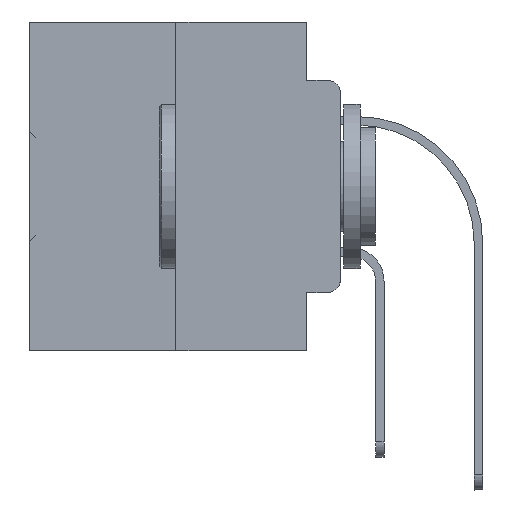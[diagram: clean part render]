
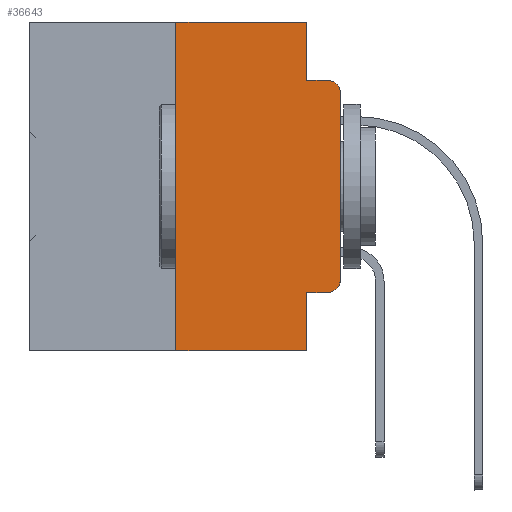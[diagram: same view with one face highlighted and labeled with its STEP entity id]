
A CAD part, left-side view. The second image highlights one B-rep face of the part: STEP entity #36643.
In plain terms, the highlighted planar face has unit normal (-1, 0, 0).
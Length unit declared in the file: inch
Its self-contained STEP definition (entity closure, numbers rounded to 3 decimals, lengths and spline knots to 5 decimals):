
#1444 = DIRECTION ( 'NONE',  ( 0., 0., -1. ) ) ;
#1654 = LINE ( 'NONE', #26141, #11457 ) ;
#1697 = CARTESIAN_POINT ( 'NONE',  ( 0., 0.473, 0. ) ) ;
#1804 = ORIENTED_EDGE ( 'NONE', *, *, #2692, .T. ) ;
#1989 = ORIENTED_EDGE ( 'NONE', *, *, #2322, .F. ) ;
#2322 = EDGE_CURVE ( 'NONE', #38294, #11469, #15991, .T. ) ;
#2692 = EDGE_CURVE ( 'NONE', #21018, #4290, #6643, .T. ) ;
#2758 = EDGE_CURVE ( 'NONE', #32369, #4290, #17079, .T. ) ;
#2951 = ORIENTED_EDGE ( 'NONE', *, *, #16692, .T. ) ;
#3166 = AXIS2_PLACEMENT_3D ( 'NONE', #30607, #5493, #18064 ) ;
#3219 = CARTESIAN_POINT ( 'NONE',  ( 0., 0., 0. ) ) ;
#3362 = CARTESIAN_POINT ( 'NONE',  ( 0., 0.473, -0.5 ) ) ;
#3396 = VECTOR ( 'NONE', #21791, 39.37008 ) ;
#3532 = EDGE_CURVE ( 'NONE', #37398, #5097, #38637, .T. ) ;
#3602 = VERTEX_POINT ( 'NONE', #37569 ) ;
#4290 = VERTEX_POINT ( 'NONE', #4984 ) ;
#4327 = DIRECTION ( 'NONE',  ( 0., -1., 0. ) ) ;
#4838 = ORIENTED_EDGE ( 'NONE', *, *, #2758, .F. ) ;
#4984 = CARTESIAN_POINT ( 'NONE',  ( 0., 0.051, -0.5 ) ) ;
#5050 = VECTOR ( 'NONE', #28550, 39.37008 ) ;
#5097 = VERTEX_POINT ( 'NONE', #39298 ) ;
#5493 = DIRECTION ( 'NONE',  ( -1., 0., 0. ) ) ;
#6643 = LINE ( 'NONE', #3362, #22549 ) ;
#7458 = DIRECTION ( 'NONE',  ( -1., 0., 0. ) ) ;
#8675 = VECTOR ( 'NONE', #28389, 39.37008 ) ;
#9003 = ORIENTED_EDGE ( 'NONE', *, *, #27369, .F. ) ;
#9231 = ORIENTED_EDGE ( 'NONE', *, *, #3532, .T. ) ;
#10164 = AXIS2_PLACEMENT_3D ( 'NONE', #32738, #7458, #32967 ) ;
#10305 = CARTESIAN_POINT ( 'NONE',  ( 0., 0., -0.1085 ) ) ;
#10973 = FACE_OUTER_BOUND ( 'NONE', #37685, .T. ) ;
#11457 = VECTOR ( 'NONE', #4327, 39.37008 ) ;
#11469 = VERTEX_POINT ( 'NONE', #20327 ) ;
#11607 = DIRECTION ( 'NONE',  ( 0., 0., -1. ) ) ;
#12340 = LINE ( 'NONE', #37397, #3396 ) ;
#12501 = LINE ( 'NONE', #3219, #33699 ) ;
#12686 = EDGE_CURVE ( 'NONE', #3602, #40446, #32276, .T. ) ;
#14261 = DIRECTION ( 'NONE',  ( 1., 0., 0. ) ) ;
#15991 = LINE ( 'NONE', #37772, #32368 ) ;
#16022 = CARTESIAN_POINT ( 'NONE',  ( 0., 0.051, 0. ) ) ;
#16301 = ORIENTED_EDGE ( 'NONE', *, *, #35863, .T. ) ;
#16537 = CARTESIAN_POINT ( 'NONE',  ( 0., 0.25, 0. ) ) ;
#16692 = EDGE_CURVE ( 'NONE', #32369, #37398, #1654, .T. ) ;
#16737 = AXIS2_PLACEMENT_3D ( 'NONE', #1697, #14261, #11607 ) ;
#17079 = LINE ( 'NONE', #29630, #17579 ) ;
#17579 = VECTOR ( 'NONE', #1444, 39.37008 ) ;
#18064 = DIRECTION ( 'NONE',  ( 0., 0., -1. ) ) ;
#18722 = CIRCLE ( 'NONE', #10164, 0.02 ) ;
#20327 = CARTESIAN_POINT ( 'NONE',  ( 0., 0.051, 0. ) ) ;
#21018 = VERTEX_POINT ( 'NONE', #34225 ) ;
#21478 = CARTESIAN_POINT ( 'NONE',  ( 0., 0.051, -0.4115 ) ) ;
#21791 = DIRECTION ( 'NONE',  ( 0., 0., 1. ) ) ;
#22549 = VECTOR ( 'NONE', #25381, 39.37008 ) ;
#22756 = DIRECTION ( 'NONE',  ( 0., -1., 0. ) ) ;
#23512 = PLANE ( 'NONE',  #16737 ) ;
#23787 = ORIENTED_EDGE ( 'NONE', *, *, #12686, .F. ) ;
#25381 = DIRECTION ( 'NONE',  ( 0., -1., 0. ) ) ;
#26141 = CARTESIAN_POINT ( 'NONE',  ( 0., 0.051, -0.4115 ) ) ;
#26958 = VERTEX_POINT ( 'NONE', #10305 ) ;
#27369 = EDGE_CURVE ( 'NONE', #21018, #38294, #12340, .T. ) ;
#28182 = CARTESIAN_POINT ( 'NONE',  ( 0., 0.051, -0.0885 ) ) ;
#28389 = DIRECTION ( 'NONE',  ( 0., -1., 0. ) ) ;
#28550 = DIRECTION ( 'NONE',  ( 0., 0., -1. ) ) ;
#29630 = CARTESIAN_POINT ( 'NONE',  ( 0., 0.051, 0. ) ) ;
#30145 = CARTESIAN_POINT ( 'NONE',  ( 0., 0.02, -0.4115 ) ) ;
#30607 = CARTESIAN_POINT ( 'NONE',  ( 0., 0.02, -0.3915 ) ) ;
#30812 = LINE ( 'NONE', #16022, #5050 ) ;
#32276 = LINE ( 'NONE', #28182, #8675 ) ;
#32368 = VECTOR ( 'NONE', #22756, 39.37008 ) ;
#32369 = VERTEX_POINT ( 'NONE', #21478 ) ;
#32738 = CARTESIAN_POINT ( 'NONE',  ( 0., 0.02, -0.1085 ) ) ;
#32967 = DIRECTION ( 'NONE',  ( 0., 0., -1. ) ) ;
#33699 = VECTOR ( 'NONE', #40472, 39.37008 ) ;
#34225 = CARTESIAN_POINT ( 'NONE',  ( 0., 0.25, -0.5 ) ) ;
#35863 = EDGE_CURVE ( 'NONE', #5097, #26958, #12501, .T. ) ;
#36555 = EDGE_CURVE ( 'NONE', #26958, #40446, #18722, .T. ) ;
#36643 = ADVANCED_FACE ( 'NONE', ( #10973 ), #23512, .F. ) ;
#37378 = ORIENTED_EDGE ( 'NONE', *, *, #36555, .T. ) ;
#37397 = CARTESIAN_POINT ( 'NONE',  ( 0., 0.25, 0. ) ) ;
#37398 = VERTEX_POINT ( 'NONE', #30145 ) ;
#37569 = CARTESIAN_POINT ( 'NONE',  ( 0., 0.051, -0.0885 ) ) ;
#37685 = EDGE_LOOP ( 'NONE', ( #16301, #37378, #23787, #39045, #1989, #9003, #1804, #4838, #2951, #9231 ) ) ;
#37772 = CARTESIAN_POINT ( 'NONE',  ( 0., 0.473, 0. ) ) ;
#38294 = VERTEX_POINT ( 'NONE', #16537 ) ;
#38463 = CARTESIAN_POINT ( 'NONE',  ( 0., 0.02, -0.0885 ) ) ;
#38637 = CIRCLE ( 'NONE', #3166, 0.02 ) ;
#39045 = ORIENTED_EDGE ( 'NONE', *, *, #40653, .F. ) ;
#39298 = CARTESIAN_POINT ( 'NONE',  ( 0., 0., -0.3915 ) ) ;
#40446 = VERTEX_POINT ( 'NONE', #38463 ) ;
#40472 = DIRECTION ( 'NONE',  ( 0., 0., 1. ) ) ;
#40653 = EDGE_CURVE ( 'NONE', #11469, #3602, #30812, .T. ) ;
